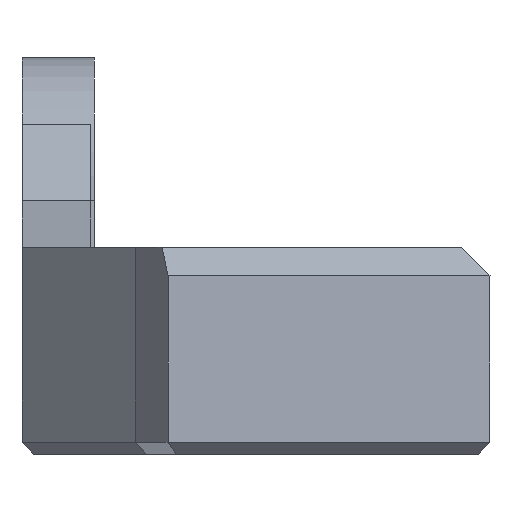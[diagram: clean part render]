
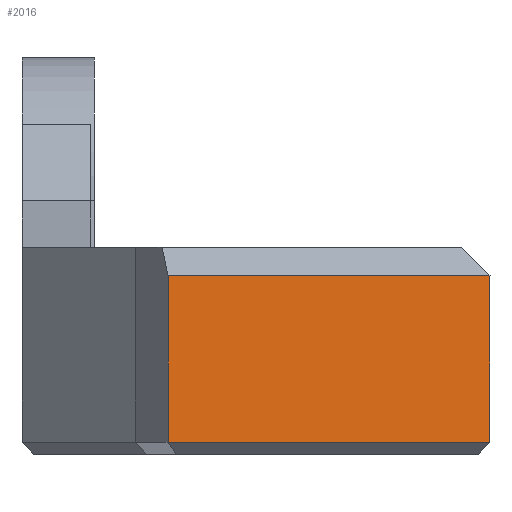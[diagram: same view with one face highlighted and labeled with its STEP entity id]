
A CAD part, left-side view. The second image highlights one B-rep face of the part: STEP entity #2016.
In plain terms, the highlighted planar face has unit normal (-0.73, -0.683, 0).
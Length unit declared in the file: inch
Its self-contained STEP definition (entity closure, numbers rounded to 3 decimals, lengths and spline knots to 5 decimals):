
#90 = DIRECTION ( 'NONE',  ( 0., 0., 1. ) ) ;
#186 = CARTESIAN_POINT ( 'NONE',  ( -4.52124, 1.198, 2.60597 ) ) ;
#271 = DIRECTION ( 'NONE',  ( -0.684, 0.73, 0. ) ) ;
#387 = ORIENTED_EDGE ( 'NONE', *, *, #891, .F. ) ;
#597 = CARTESIAN_POINT ( 'NONE',  ( -4.92154, 1.62549, 4.05299 ) ) ;
#781 = VECTOR ( 'NONE', #90, 39.37008 ) ;
#891 = EDGE_CURVE ( 'NONE', #1957, #2448, #2385, .T. ) ;
#1034 = VERTEX_POINT ( 'NONE', #186 ) ;
#1059 = LINE ( 'NONE', #3855, #3545 ) ;
#1154 = FACE_OUTER_BOUND ( 'NONE', #1313, .T. ) ;
#1176 = PLANE ( 'NONE',  #3520 ) ;
#1227 = VERTEX_POINT ( 'NONE', #2756 ) ;
#1313 = EDGE_LOOP ( 'NONE', ( #387, #2309, #2225, #1492 ) ) ;
#1376 = LINE ( 'NONE', #3767, #3640 ) ;
#1423 = VECTOR ( 'NONE', #3811, 39.37008 ) ;
#1492 = ORIENTED_EDGE ( 'NONE', *, *, #2026, .T. ) ;
#1947 = EDGE_CURVE ( 'NONE', #1034, #1227, #2654, .T. ) ;
#1957 = VERTEX_POINT ( 'NONE', #3782 ) ;
#2016 = ADVANCED_FACE ( 'NONE', ( #1154 ), #1176, .T. ) ;
#2026 = EDGE_CURVE ( 'NONE', #1034, #2448, #1059, .T. ) ;
#2184 = CARTESIAN_POINT ( 'NONE',  ( -4.91753, 1.6212, 4.05299 ) ) ;
#2215 = EDGE_CURVE ( 'NONE', #1957, #1227, #1376, .T. ) ;
#2225 = ORIENTED_EDGE ( 'NONE', *, *, #1947, .F. ) ;
#2309 = ORIENTED_EDGE ( 'NONE', *, *, #2215, .T. ) ;
#2385 = LINE ( 'NONE', #2184, #781 ) ;
#2448 = VERTEX_POINT ( 'NONE', #3074 ) ;
#2654 = LINE ( 'NONE', #3471, #1423 ) ;
#2661 = DIRECTION ( 'NONE',  ( -0.73, -0.684, 0. ) ) ;
#2756 = CARTESIAN_POINT ( 'NONE',  ( -4.52124, 1.198, 2.38722 ) ) ;
#2888 = DIRECTION ( 'NONE',  ( 0.684, -0.73, 0. ) ) ;
#3074 = CARTESIAN_POINT ( 'NONE',  ( -4.91753, 1.6212, 2.60597 ) ) ;
#3471 = CARTESIAN_POINT ( 'NONE',  ( -4.52124, 1.198, 4.05299 ) ) ;
#3520 = AXIS2_PLACEMENT_3D ( 'NONE', #597, #2661, #3563 ) ;
#3545 = VECTOR ( 'NONE', #271, 39.37008 ) ;
#3563 = DIRECTION ( 'NONE',  ( 0.684, -0.73, 0. ) ) ;
#3640 = VECTOR ( 'NONE', #2888, 39.37008 ) ;
#3767 = CARTESIAN_POINT ( 'NONE',  ( -4.52124, 1.198, 2.38722 ) ) ;
#3782 = CARTESIAN_POINT ( 'NONE',  ( -4.91753, 1.6212, 2.38722 ) ) ;
#3811 = DIRECTION ( 'NONE',  ( 0., 0., -1. ) ) ;
#3855 = CARTESIAN_POINT ( 'NONE',  ( -4.92154, 1.62549, 2.60597 ) ) ;
